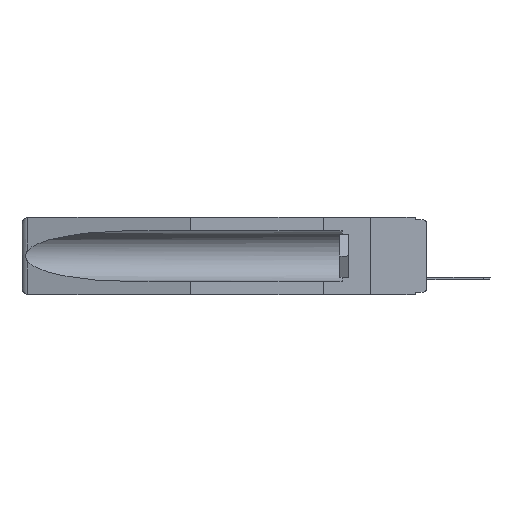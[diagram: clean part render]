
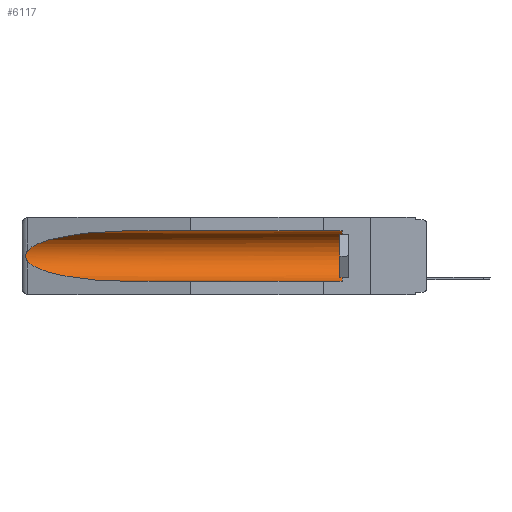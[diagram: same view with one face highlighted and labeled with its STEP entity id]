
A CAD part, left-side view. The second image highlights one B-rep face of the part: STEP entity #6117.
In plain terms, the highlighted cylindrical face has radius 2.857 mm (diameter 5.715 mm), a partial arc.
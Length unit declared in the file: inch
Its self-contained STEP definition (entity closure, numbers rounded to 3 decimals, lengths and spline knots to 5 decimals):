
#777 = CARTESIAN_POINT ( 'NONE',  ( 0.26597, 1.5296, -0.19026 ) ) ;
#1466 = CARTESIAN_POINT ( 'NONE',  ( 0.155, 0.126, -0.284 ) ) ;
#1573 = CARTESIAN_POINT ( 'NONE',  ( 0.25451, 1.48313, -0.24835 ) ) ;
#1744 = VECTOR ( 'NONE', #15459, 39.37008 ) ;
#2291 = ORIENTED_EDGE ( 'NONE', *, *, #11184, .T. ) ;
#2686 = DIRECTION ( 'NONE',  ( 0., 0., 1. ) ) ;
#2844 = EDGE_CURVE ( 'NONE', #5673, #8918, #5540, .T. ) ;
#3379 = CARTESIAN_POINT ( 'NONE',  ( 0.155, 1.07973, -0.059 ) ) ;
#3797 = ORIENTED_EDGE ( 'NONE', *, *, #10343, .F. ) ;
#3814 =( BOUNDED_CURVE ( )  B_SPLINE_CURVE ( 3, ( #3379, #9627, #14721, #7179 ),
 .UNSPECIFIED., .F., .T. ) 
 B_SPLINE_CURVE_WITH_KNOTS ( ( 4, 4 ),
 ( 4.71239, 6.08839 ),
 .UNSPECIFIED. ) 
 CURVE ( )  GEOMETRIC_REPRESENTATION_ITEM ( )  RATIONAL_B_SPLINE_CURVE ( ( 1., 0.848, 0.848, 1. ) ) 
 REPRESENTATION_ITEM ( '' )  );
#4386 = CARTESIAN_POINT ( 'NONE',  ( 0.26655, 1.53094, -0.18657 ) ) ;
#4423 = DIRECTION ( 'NONE',  ( 0., 1., 0. ) ) ;
#4468 = CARTESIAN_POINT ( 'NONE',  ( 0.2675, 1.53308, -0.16763 ) ) ;
#4495 = DIRECTION ( 'NONE',  ( 0., 0., 1. ) ) ;
#4509 = ORIENTED_EDGE ( 'NONE', *, *, #12458, .T. ) ;
#4548 = CARTESIAN_POINT ( 'NONE',  ( 0.2673, 1.53269, -0.17917 ) ) ;
#4570 = CYLINDRICAL_SURFACE ( 'NONE', #14646, 0.1125 ) ;
#4794 = CARTESIAN_POINT ( 'NONE',  ( 0.155, -0.30754, -0.1715 ) ) ;
#4837 = VECTOR ( 'NONE', #4423, 39.37008 ) ;
#5057 =( BOUNDED_CURVE ( )  B_SPLINE_CURVE ( 3, ( #9164, #1573, #13010, #10638 ),
 .UNSPECIFIED., .F., .T. ) 
 B_SPLINE_CURVE_WITH_KNOTS ( ( 4, 4 ),
 ( 0.1948, 1.5708 ),
 .UNSPECIFIED. ) 
 CURVE ( )  GEOMETRIC_REPRESENTATION_ITEM ( )  RATIONAL_B_SPLINE_CURVE ( ( 1., 0.848, 0.848, 1. ) ) 
 REPRESENTATION_ITEM ( '' )  );
#5540 = CIRCLE ( 'NONE', #13758, 0.1125 ) ;
#5673 = VERTEX_POINT ( 'NONE', #1466 ) ;
#5766 = CARTESIAN_POINT ( 'NONE',  ( 0.26537, 1.52718, -0.14972 ) ) ;
#6041 = LINE ( 'NONE', #10739, #4837 ) ;
#6117 = ADVANCED_FACE ( 'NONE', ( #15837 ), #4570, .F. ) ;
#7179 = CARTESIAN_POINT ( 'NONE',  ( 0.26537, 1.52718, -0.14972 ) ) ;
#7328 = EDGE_CURVE ( 'NONE', #7353, #14340, #5057, .T. ) ;
#7353 = VERTEX_POINT ( 'NONE', #9406 ) ;
#7444 = CARTESIAN_POINT ( 'NONE',  ( 0.155, 0.126, -0.059 ) ) ;
#7949 = VERTEX_POINT ( 'NONE', #15907 ) ;
#8120 = CARTESIAN_POINT ( 'NONE',  ( 0.155, 1.07973, -0.284 ) ) ;
#8317 = CARTESIAN_POINT ( 'NONE',  ( 0.2675, 1.53308, -0.17534 ) ) ;
#8800 = DIRECTION ( 'NONE',  ( 0., -1., 0. ) ) ;
#8918 = VERTEX_POINT ( 'NONE', #7444 ) ;
#9164 = CARTESIAN_POINT ( 'NONE',  ( 0.26537, 1.52718, -0.19328 ) ) ;
#9406 = CARTESIAN_POINT ( 'NONE',  ( 0.26537, 1.52718, -0.19328 ) ) ;
#9455 = LINE ( 'NONE', #10347, #1744 ) ;
#9627 = CARTESIAN_POINT ( 'NONE',  ( 0.21114, 1.30732, -0.059 ) ) ;
#10329 = EDGE_LOOP ( 'NONE', ( #4509, #2291, #11842, #3797, #13242, #13263 ) ) ;
#10343 = EDGE_CURVE ( 'NONE', #5673, #14340, #6041, .T. ) ;
#10347 = CARTESIAN_POINT ( 'NONE',  ( 0.155, -0.30754, -0.059 ) ) ;
#10419 = VERTEX_POINT ( 'NONE', #13517 ) ;
#10638 = CARTESIAN_POINT ( 'NONE',  ( 0.155, 1.07973, -0.284 ) ) ;
#10739 = CARTESIAN_POINT ( 'NONE',  ( 0.155, -0.30754, -0.284 ) ) ;
#10782 = CARTESIAN_POINT ( 'NONE',  ( 0.26654, 1.53092, -0.15636 ) ) ;
#10862 = CARTESIAN_POINT ( 'NONE',  ( 0.26597, 1.52961, -0.15275 ) ) ;
#10963 = DIRECTION ( 'NONE',  ( 0., 1., 0. ) ) ;
#11184 = EDGE_CURVE ( 'NONE', #7949, #7353, #16339, .T. ) ;
#11198 = CARTESIAN_POINT ( 'NONE',  ( 0.155, 0.126, -0.1715 ) ) ;
#11842 = ORIENTED_EDGE ( 'NONE', *, *, #7328, .T. ) ;
#11956 = CARTESIAN_POINT ( 'NONE',  ( 0.26537, 1.52718, -0.19328 ) ) ;
#12458 = EDGE_CURVE ( 'NONE', #10419, #7949, #3814, .T. ) ;
#13010 = CARTESIAN_POINT ( 'NONE',  ( 0.21114, 1.30732, -0.284 ) ) ;
#13242 = ORIENTED_EDGE ( 'NONE', *, *, #2844, .T. ) ;
#13263 = ORIENTED_EDGE ( 'NONE', *, *, #15688, .T. ) ;
#13517 = CARTESIAN_POINT ( 'NONE',  ( 0.155, 1.07973, -0.059 ) ) ;
#13758 = AXIS2_PLACEMENT_3D ( 'NONE', #11198, #8800, #2686 ) ;
#14340 = VERTEX_POINT ( 'NONE', #8120 ) ;
#14646 = AXIS2_PLACEMENT_3D ( 'NONE', #4794, #10963, #4495 ) ;
#14721 = CARTESIAN_POINT ( 'NONE',  ( 0.25451, 1.48313, -0.09465 ) ) ;
#15459 = DIRECTION ( 'NONE',  ( 0., 1., 0. ) ) ;
#15688 = EDGE_CURVE ( 'NONE', #8918, #10419, #9455, .T. ) ;
#15837 = FACE_OUTER_BOUND ( 'NONE', #10329, .T. ) ;
#15898 = CARTESIAN_POINT ( 'NONE',  ( 0.2673, 1.5327, -0.16383 ) ) ;
#15907 = CARTESIAN_POINT ( 'NONE',  ( 0.26537, 1.52718, -0.14972 ) ) ;
#16339 = B_SPLINE_CURVE_WITH_KNOTS ( 'NONE', 3,
 ( #5766, #10862, #10782, #15898, #4468, #8317, #4548, #4386, #777, #11956 ),
 .UNSPECIFIED., .F., .F.,
 ( 4, 2, 2, 2, 4 ),
 ( 0., 0.00029, 0.00058, 0.00087, 0.00117 ),
 .UNSPECIFIED. ) ;
